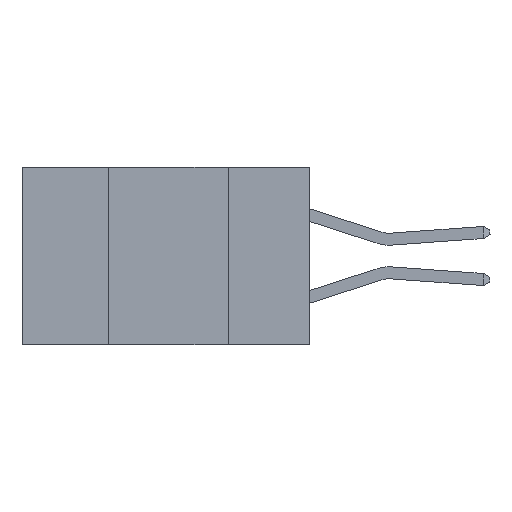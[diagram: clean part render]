
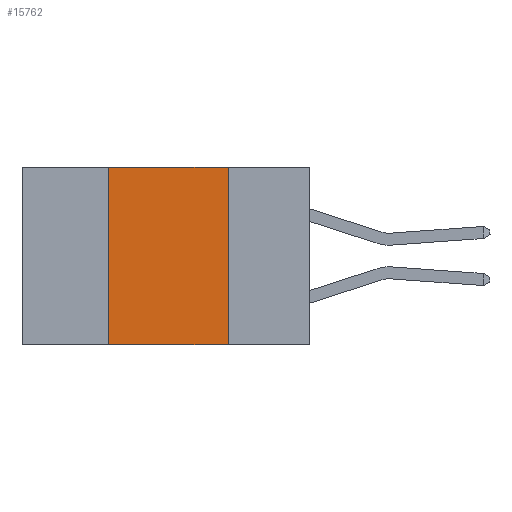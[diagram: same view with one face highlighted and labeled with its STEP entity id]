
A CAD part, left-side view. The second image highlights one B-rep face of the part: STEP entity #15762.
In plain terms, the highlighted planar face has unit normal (-1, 0, 0).
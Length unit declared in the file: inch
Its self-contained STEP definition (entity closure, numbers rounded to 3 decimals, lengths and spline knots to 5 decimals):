
#28 = VERTEX_POINT ( 'NONE', #5161 ) ;
#172 = ORIENTED_EDGE ( 'NONE', *, *, #8793, .F. ) ;
#825 = EDGE_LOOP ( 'NONE', ( #8327, #172, #5576, #5190 ) ) ;
#1761 = DIRECTION ( 'NONE',  ( 0., -1., 0. ) ) ;
#1849 = DIRECTION ( 'NONE',  ( 1., 0., 0. ) ) ;
#1908 = CARTESIAN_POINT ( 'NONE',  ( 0., 0.6, -0.37 ) ) ;
#2649 = CARTESIAN_POINT ( 'NONE',  ( 0., 0.6, 0. ) ) ;
#2672 = DIRECTION ( 'NONE',  ( 0., -1., 0. ) ) ;
#3599 = FACE_OUTER_BOUND ( 'NONE', #825, .T. ) ;
#3792 = LINE ( 'NONE', #13118, #13378 ) ;
#5161 = CARTESIAN_POINT ( 'NONE',  ( 0., 0.42, -0.37 ) ) ;
#5190 = ORIENTED_EDGE ( 'NONE', *, *, #8255, .T. ) ;
#5576 = ORIENTED_EDGE ( 'NONE', *, *, #8941, .F. ) ;
#6168 = VECTOR ( 'NONE', #1761, 39.37008 ) ;
#6440 = AXIS2_PLACEMENT_3D ( 'NONE', #13329, #1849, #7363 ) ;
#7363 = DIRECTION ( 'NONE',  ( 0., 0., -1. ) ) ;
#7670 = CARTESIAN_POINT ( 'NONE',  ( 0., 0.42, 0. ) ) ;
#8255 = EDGE_CURVE ( 'NONE', #28, #11493, #9709, .T. ) ;
#8327 = ORIENTED_EDGE ( 'NONE', *, *, #9051, .F. ) ;
#8793 = EDGE_CURVE ( 'NONE', #11178, #13266, #9875, .T. ) ;
#8863 = VECTOR ( 'NONE', #12313, 39.37008 ) ;
#8941 = EDGE_CURVE ( 'NONE', #28, #11178, #3792, .T. ) ;
#9051 = EDGE_CURVE ( 'NONE', #13266, #11493, #9293, .T. ) ;
#9293 = LINE ( 'NONE', #12327, #8863 ) ;
#9709 = LINE ( 'NONE', #1908, #6168 ) ;
#9875 = LINE ( 'NONE', #2649, #15619 ) ;
#11178 = VERTEX_POINT ( 'NONE', #7670 ) ;
#11493 = VERTEX_POINT ( 'NONE', #13107 ) ;
#12313 = DIRECTION ( 'NONE',  ( 0., 0., -1. ) ) ;
#12327 = CARTESIAN_POINT ( 'NONE',  ( 0., 0.17, -0.37 ) ) ;
#13078 = DIRECTION ( 'NONE',  ( 0., 0., 1. ) ) ;
#13107 = CARTESIAN_POINT ( 'NONE',  ( 0., 0.17, -0.37 ) ) ;
#13118 = CARTESIAN_POINT ( 'NONE',  ( 0., 0.42, -0.37 ) ) ;
#13266 = VERTEX_POINT ( 'NONE', #15917 ) ;
#13329 = CARTESIAN_POINT ( 'NONE',  ( 0., 0.6, 0. ) ) ;
#13378 = VECTOR ( 'NONE', #13078, 39.37008 ) ;
#14386 = PLANE ( 'NONE',  #6440 ) ;
#15619 = VECTOR ( 'NONE', #2672, 39.37008 ) ;
#15762 = ADVANCED_FACE ( 'NONE', ( #3599 ), #14386, .F. ) ;
#15917 = CARTESIAN_POINT ( 'NONE',  ( 0., 0.17, 0. ) ) ;
